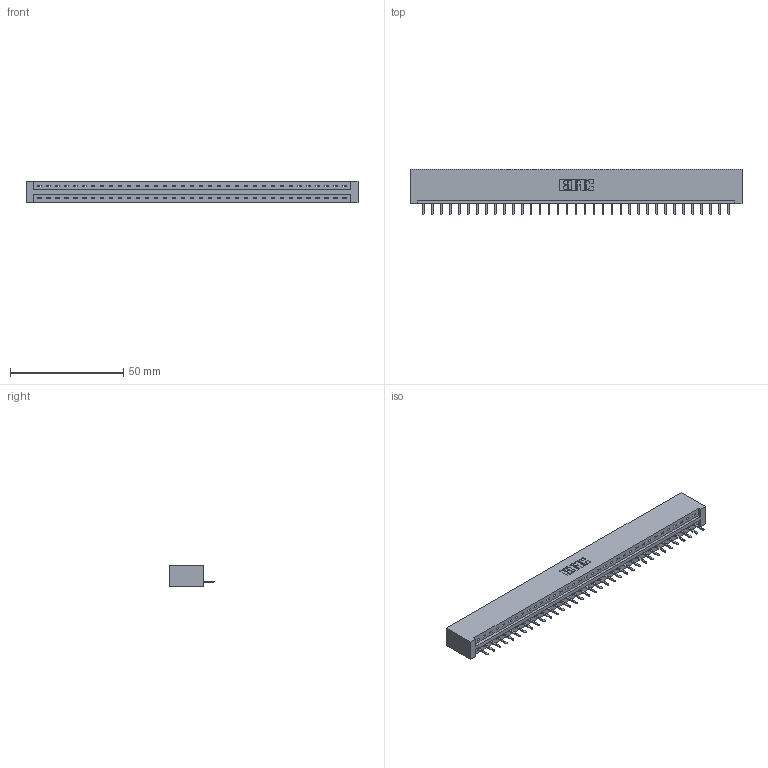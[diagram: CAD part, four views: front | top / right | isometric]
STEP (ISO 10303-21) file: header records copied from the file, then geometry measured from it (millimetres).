
FILE_DESCRIPTION (( 'STEP AP203' ), '1' );
FILE_NAME ('337-035-520-101.STEP', '2019-10-01T12:26:58', ( '' ), ( '' ), 'SwSTEP 2.0', 'SolidWorks 2016', '' );
FILE_SCHEMA (( 'CONFIG_CONTROL_DESIGN' ));
Length unit declared in the file: inch
Products named in the file (3): 337-035-520-101; 345-292-001_345-293-120; 337 Part_No Mounting Lugs
Assembly tree (36 placements, depth 2):
  337-035-520-101
    337 Part_No Mounting Lugs
    345-292-001_345-293-120  x35
Bounding box: 146.56 x 20.02 x 9.4 mm (x, y, z)
Volume: 15782.7 mm3; surface area: 15889.3 mm2
Topology: 36 solids, 36 shells, 2416 faces, 7147 edges, 4670 vertices
Faces by surface type: plane 1746, cylinder 670
Entity records: 26759 total; most frequent: CARTESIAN_POINT 4679, ORIENTED_EDGE 4638, DIRECTION 3933, EDGE_CURVE 2319, VECTOR 2195, LINE 2195, VERTEX_POINT 1542, AXIS2_PLACEMENT_3D 869
